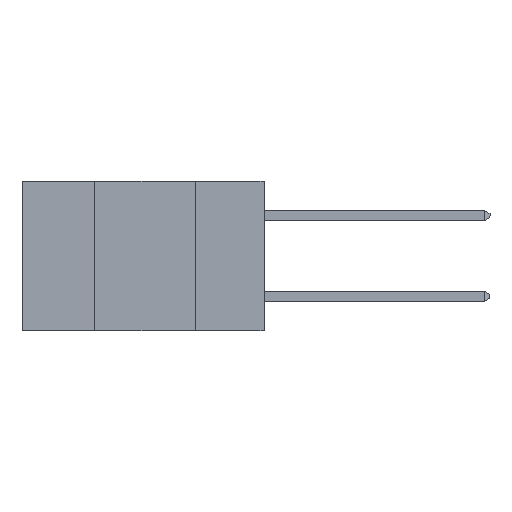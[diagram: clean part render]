
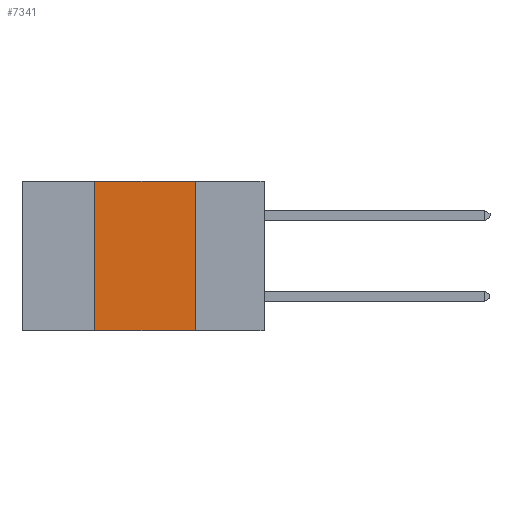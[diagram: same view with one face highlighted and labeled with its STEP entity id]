
A CAD part, left-side view. The second image highlights one B-rep face of the part: STEP entity #7341.
In plain terms, the highlighted planar face has unit normal (-1, 0, 0).
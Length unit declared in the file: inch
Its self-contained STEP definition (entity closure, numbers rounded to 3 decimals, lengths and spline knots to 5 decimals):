
#163 = DIRECTION ( 'NONE',  ( 0., 0., -1. ) ) ;
#1000 = LINE ( 'NONE', #7329, #12184 ) ;
#1473 = CARTESIAN_POINT ( 'NONE',  ( 0., 0.17, 0. ) ) ;
#1770 = DIRECTION ( 'NONE',  ( 0., 0., -1. ) ) ;
#2223 = VERTEX_POINT ( 'NONE', #4169 ) ;
#2309 = CARTESIAN_POINT ( 'NONE',  ( 0., 0.6, 0. ) ) ;
#3216 = VECTOR ( 'NONE', #5926, 39.37008 ) ;
#3840 = ORIENTED_EDGE ( 'NONE', *, *, #6406, .F. ) ;
#3905 = ORIENTED_EDGE ( 'NONE', *, *, #5544, .F. ) ;
#4097 = EDGE_CURVE ( 'NONE', #8781, #11563, #6282, .T. ) ;
#4169 = CARTESIAN_POINT ( 'NONE',  ( 0., 0.42, 0. ) ) ;
#4201 = ORIENTED_EDGE ( 'NONE', *, *, #5636, .F. ) ;
#4244 = ORIENTED_EDGE ( 'NONE', *, *, #4097, .T. ) ;
#4307 = CARTESIAN_POINT ( 'NONE',  ( 0., 0.42, -0.37 ) ) ;
#4422 = VECTOR ( 'NONE', #13419, 39.37008 ) ;
#4931 = VERTEX_POINT ( 'NONE', #1473 ) ;
#5544 = EDGE_CURVE ( 'NONE', #2223, #4931, #8825, .T. ) ;
#5636 = EDGE_CURVE ( 'NONE', #8781, #2223, #10576, .T. ) ;
#5905 = AXIS2_PLACEMENT_3D ( 'NONE', #2309, #6833, #163 ) ;
#5926 = DIRECTION ( 'NONE',  ( 0., -1., 0. ) ) ;
#6282 = LINE ( 'NONE', #13183, #6639 ) ;
#6406 = EDGE_CURVE ( 'NONE', #4931, #11563, #1000, .T. ) ;
#6639 = VECTOR ( 'NONE', #13629, 39.37008 ) ;
#6833 = DIRECTION ( 'NONE',  ( 1., 0., 0. ) ) ;
#7329 = CARTESIAN_POINT ( 'NONE',  ( 0., 0.17, 0. ) ) ;
#7341 = ADVANCED_FACE ( 'NONE', ( #8110 ), #12067, .F. ) ;
#8110 = FACE_OUTER_BOUND ( 'NONE', #13541, .T. ) ;
#8315 = CARTESIAN_POINT ( 'NONE',  ( 0., 0.42, 0. ) ) ;
#8781 = VERTEX_POINT ( 'NONE', #4307 ) ;
#8825 = LINE ( 'NONE', #13289, #3216 ) ;
#10576 = LINE ( 'NONE', #8315, #4422 ) ;
#11563 = VERTEX_POINT ( 'NONE', #13533 ) ;
#12067 = PLANE ( 'NONE',  #5905 ) ;
#12184 = VECTOR ( 'NONE', #1770, 39.37008 ) ;
#13183 = CARTESIAN_POINT ( 'NONE',  ( 0., 0.6, -0.37 ) ) ;
#13289 = CARTESIAN_POINT ( 'NONE',  ( 0., 0.6, 0. ) ) ;
#13419 = DIRECTION ( 'NONE',  ( 0., 0., 1. ) ) ;
#13533 = CARTESIAN_POINT ( 'NONE',  ( 0., 0.17, -0.37 ) ) ;
#13541 = EDGE_LOOP ( 'NONE', ( #3840, #3905, #4201, #4244 ) ) ;
#13629 = DIRECTION ( 'NONE',  ( 0., -1., 0. ) ) ;
